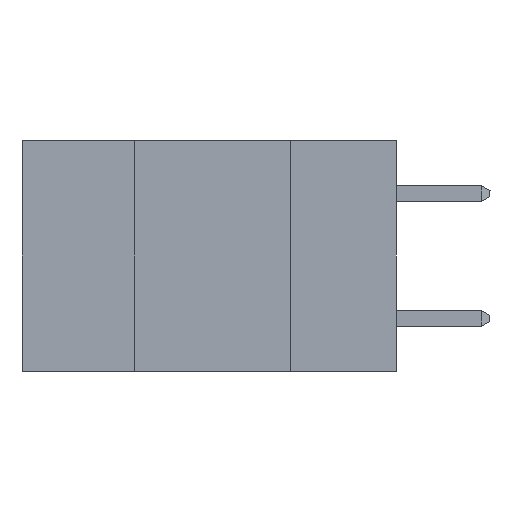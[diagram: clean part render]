
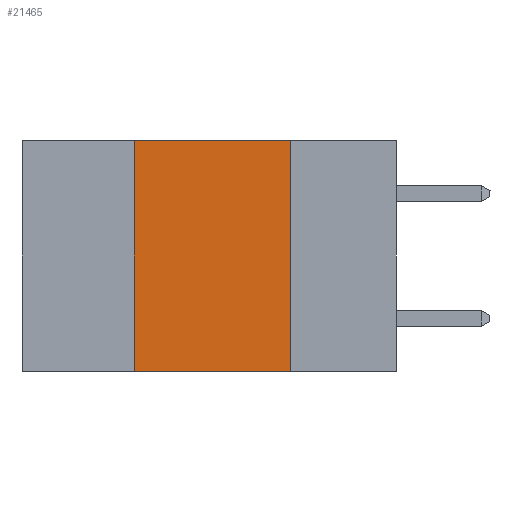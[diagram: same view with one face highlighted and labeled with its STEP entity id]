
A CAD part, left-side view. The second image highlights one B-rep face of the part: STEP entity #21465.
In plain terms, the highlighted planar face has unit normal (-1, 0, 0).
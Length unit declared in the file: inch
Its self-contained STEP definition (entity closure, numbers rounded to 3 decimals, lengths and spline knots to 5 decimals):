
#64 = LINE ( 'NONE', #2186, #21924 ) ;
#716 = EDGE_LOOP ( 'NONE', ( #11901, #21090, #9888, #3571 ) ) ;
#1187 = CARTESIAN_POINT ( 'NONE',  ( 0., 0.42, -0.37 ) ) ;
#1804 = LINE ( 'NONE', #23161, #18065 ) ;
#2156 = DIRECTION ( 'NONE',  ( 0., -1., 0. ) ) ;
#2186 = CARTESIAN_POINT ( 'NONE',  ( 0., 0.17, -0.37 ) ) ;
#2428 = DIRECTION ( 'NONE',  ( 0., -1., 0. ) ) ;
#3478 = EDGE_CURVE ( 'NONE', #10129, #5714, #6681, .T. ) ;
#3571 = ORIENTED_EDGE ( 'NONE', *, *, #3478, .T. ) ;
#4113 = AXIS2_PLACEMENT_3D ( 'NONE', #13333, #19632, #6964 ) ;
#4345 = DIRECTION ( 'NONE',  ( 0., 0., -1. ) ) ;
#5714 = VERTEX_POINT ( 'NONE', #6183 ) ;
#6183 = CARTESIAN_POINT ( 'NONE',  ( 0., 0.17, -0.37 ) ) ;
#6607 = CARTESIAN_POINT ( 'NONE',  ( 0., 0.6, -0.37 ) ) ;
#6681 = LINE ( 'NONE', #6607, #22805 ) ;
#6964 = DIRECTION ( 'NONE',  ( 0., 0., -1. ) ) ;
#9660 = DIRECTION ( 'NONE',  ( 0., 0., 1. ) ) ;
#9888 = ORIENTED_EDGE ( 'NONE', *, *, #10595, .F. ) ;
#10129 = VERTEX_POINT ( 'NONE', #16815 ) ;
#10595 = EDGE_CURVE ( 'NONE', #10129, #12421, #24269, .T. ) ;
#10793 = CARTESIAN_POINT ( 'NONE',  ( 0., 0.17, 0. ) ) ;
#11901 = ORIENTED_EDGE ( 'NONE', *, *, #13444, .F. ) ;
#12012 = EDGE_CURVE ( 'NONE', #12421, #26120, #1804, .T. ) ;
#12421 = VERTEX_POINT ( 'NONE', #26169 ) ;
#13073 = FACE_OUTER_BOUND ( 'NONE', #716, .T. ) ;
#13333 = CARTESIAN_POINT ( 'NONE',  ( 0., 0.6, 0. ) ) ;
#13444 = EDGE_CURVE ( 'NONE', #26120, #5714, #64, .T. ) ;
#13871 = VECTOR ( 'NONE', #9660, 39.37008 ) ;
#16815 = CARTESIAN_POINT ( 'NONE',  ( 0., 0.42, -0.37 ) ) ;
#18065 = VECTOR ( 'NONE', #2156, 39.37008 ) ;
#19632 = DIRECTION ( 'NONE',  ( 1., 0., 0. ) ) ;
#21090 = ORIENTED_EDGE ( 'NONE', *, *, #12012, .F. ) ;
#21465 = ADVANCED_FACE ( 'NONE', ( #13073 ), #25763, .F. ) ;
#21924 = VECTOR ( 'NONE', #4345, 39.37008 ) ;
#22805 = VECTOR ( 'NONE', #2428, 39.37008 ) ;
#23161 = CARTESIAN_POINT ( 'NONE',  ( 0., 0.6, 0. ) ) ;
#24269 = LINE ( 'NONE', #1187, #13871 ) ;
#25763 = PLANE ( 'NONE',  #4113 ) ;
#26120 = VERTEX_POINT ( 'NONE', #10793 ) ;
#26169 = CARTESIAN_POINT ( 'NONE',  ( 0., 0.42, 0. ) ) ;
